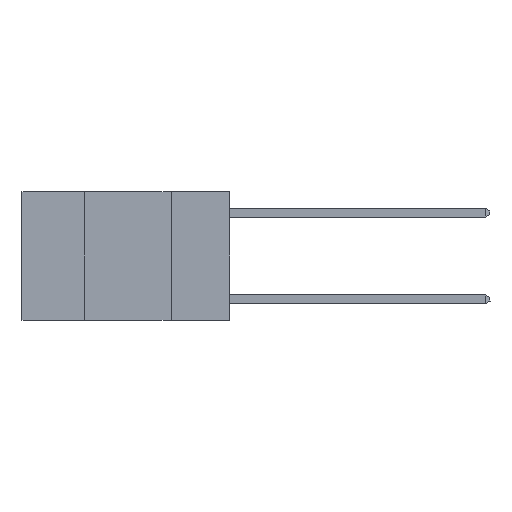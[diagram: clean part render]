
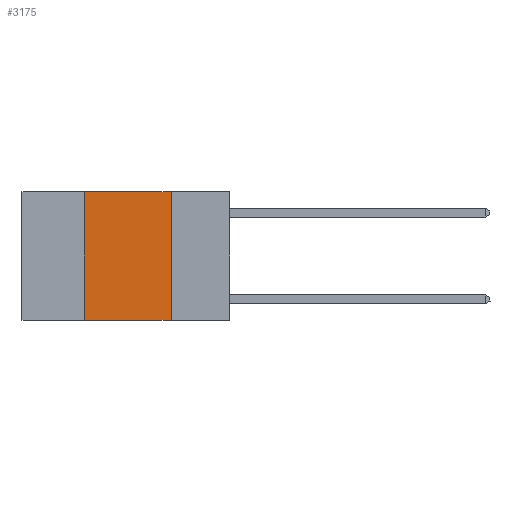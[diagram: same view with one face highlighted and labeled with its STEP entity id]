
A CAD part, left-side view. The second image highlights one B-rep face of the part: STEP entity #3175.
In plain terms, the highlighted planar face has unit normal (-1, 0, 0).
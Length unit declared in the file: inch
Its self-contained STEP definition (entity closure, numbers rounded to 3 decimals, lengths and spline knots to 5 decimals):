
#12 = VECTOR ( 'NONE', #4801, 39.37008 ) ;
#96 = CARTESIAN_POINT ( 'NONE',  ( 0., 0.17, -0.37 ) ) ;
#126 = VERTEX_POINT ( 'NONE', #625 ) ;
#414 = DIRECTION ( 'NONE',  ( 0., -1., 0. ) ) ;
#625 = CARTESIAN_POINT ( 'NONE',  ( 0., 0.42, 0. ) ) ;
#644 = DIRECTION ( 'NONE',  ( 0., 0., -1. ) ) ;
#647 = DIRECTION ( 'NONE',  ( 0., -1., 0. ) ) ;
#658 = ORIENTED_EDGE ( 'NONE', *, *, #4439, .F. ) ;
#1220 = EDGE_CURVE ( 'NONE', #3305, #2882, #5100, .T. ) ;
#1899 = VECTOR ( 'NONE', #414, 39.37008 ) ;
#2604 = EDGE_CURVE ( 'NONE', #9301, #2882, #4123, .T. ) ;
#2710 = ORIENTED_EDGE ( 'NONE', *, *, #9515, .F. ) ;
#2722 = DIRECTION ( 'NONE',  ( 0., 0., -1. ) ) ;
#2870 = AXIS2_PLACEMENT_3D ( 'NONE', #4946, #5762, #2722 ) ;
#2882 = VERTEX_POINT ( 'NONE', #96 ) ;
#3175 = ADVANCED_FACE ( 'NONE', ( #5453 ), #4560, .F. ) ;
#3305 = VERTEX_POINT ( 'NONE', #5067 ) ;
#3874 = EDGE_LOOP ( 'NONE', ( #8446, #658, #2710, #8676 ) ) ;
#4123 = LINE ( 'NONE', #7361, #1899 ) ;
#4336 = LINE ( 'NONE', #8536, #12 ) ;
#4400 = CARTESIAN_POINT ( 'NONE',  ( 0., 0.6, 0. ) ) ;
#4439 = EDGE_CURVE ( 'NONE', #126, #3305, #8955, .T. ) ;
#4560 = PLANE ( 'NONE',  #2870 ) ;
#4621 = VECTOR ( 'NONE', #644, 39.37008 ) ;
#4801 = DIRECTION ( 'NONE',  ( 0., 0., 1. ) ) ;
#4946 = CARTESIAN_POINT ( 'NONE',  ( 0., 0.6, 0. ) ) ;
#5067 = CARTESIAN_POINT ( 'NONE',  ( 0., 0.17, 0. ) ) ;
#5100 = LINE ( 'NONE', #7901, #4621 ) ;
#5453 = FACE_OUTER_BOUND ( 'NONE', #3874, .T. ) ;
#5762 = DIRECTION ( 'NONE',  ( 1., 0., 0. ) ) ;
#6720 = VECTOR ( 'NONE', #647, 39.37008 ) ;
#7361 = CARTESIAN_POINT ( 'NONE',  ( 0., 0.6, -0.37 ) ) ;
#7901 = CARTESIAN_POINT ( 'NONE',  ( 0., 0.17, 0. ) ) ;
#8446 = ORIENTED_EDGE ( 'NONE', *, *, #1220, .F. ) ;
#8536 = CARTESIAN_POINT ( 'NONE',  ( 0., 0.42, 0. ) ) ;
#8676 = ORIENTED_EDGE ( 'NONE', *, *, #2604, .T. ) ;
#8955 = LINE ( 'NONE', #4400, #6720 ) ;
#9059 = CARTESIAN_POINT ( 'NONE',  ( 0., 0.42, -0.37 ) ) ;
#9301 = VERTEX_POINT ( 'NONE', #9059 ) ;
#9515 = EDGE_CURVE ( 'NONE', #9301, #126, #4336, .T. ) ;
